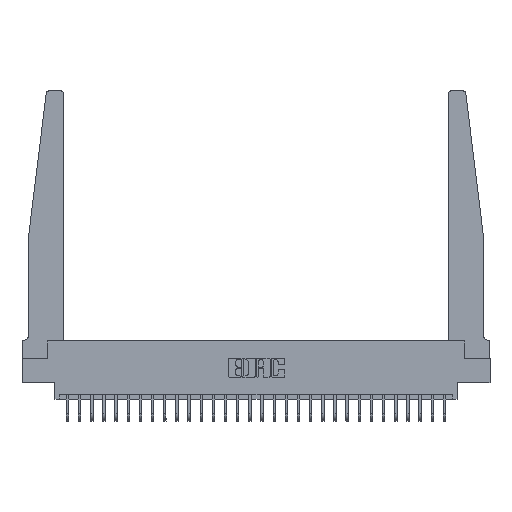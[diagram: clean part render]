
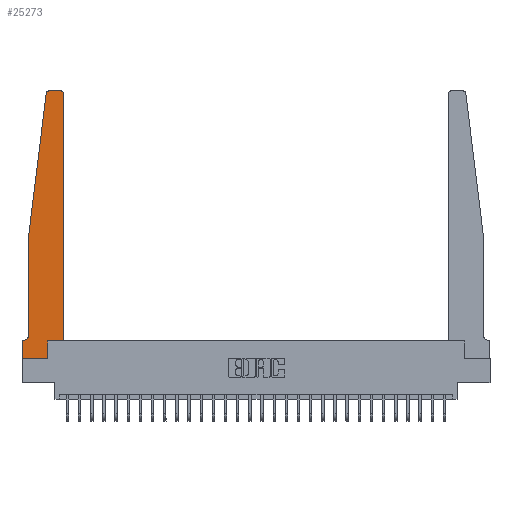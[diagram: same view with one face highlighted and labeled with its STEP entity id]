
A CAD part, top view. The second image highlights one B-rep face of the part: STEP entity #25273.
In plain terms, the highlighted planar face has unit normal (0, 0, 1).
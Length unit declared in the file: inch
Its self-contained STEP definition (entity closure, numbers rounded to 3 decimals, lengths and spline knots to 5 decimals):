
#40 = ORIENTED_EDGE ( 'NONE', *, *, #7844, .T. ) ;
#221 = VECTOR ( 'NONE', #22805, 39.37008 ) ;
#355 = EDGE_CURVE ( 'NONE', #20251, #21731, #25838, .T. ) ;
#581 = CARTESIAN_POINT ( 'NONE',  ( 0.2605, 0.18, 0.37 ) ) ;
#600 = EDGE_CURVE ( 'NONE', #10859, #20251, #25806, .T. ) ;
#1405 = VERTEX_POINT ( 'NONE', #17581 ) ;
#1529 = EDGE_CURVE ( 'NONE', #1405, #14555, #12156, .T. ) ;
#2232 = AXIS2_PLACEMENT_3D ( 'NONE', #16033, #5373, #23232 ) ;
#3076 = CARTESIAN_POINT ( 'NONE',  ( 0.24675, 2.72367, 0.37 ) ) ;
#4042 = VERTEX_POINT ( 'NONE', #8769 ) ;
#4083 = EDGE_CURVE ( 'NONE', #18692, #12985, #16721, .T. ) ;
#4384 = ORIENTED_EDGE ( 'NONE', *, *, #1529, .T. ) ;
#4479 = CARTESIAN_POINT ( 'NONE',  ( 0.425, 0.18, 0.37 ) ) ;
#4892 = CARTESIAN_POINT ( 'NONE',  ( 0.2605, 0., 0.37 ) ) ;
#5170 = DIRECTION ( 'NONE',  ( 0., -1., 0. ) ) ;
#5373 = DIRECTION ( 'NONE',  ( 0., 0., 1. ) ) ;
#6184 = ORIENTED_EDGE ( 'NONE', *, *, #24837, .T. ) ;
#6224 = DIRECTION ( 'NONE',  ( -1., 0., 0. ) ) ;
#6511 = VERTEX_POINT ( 'NONE', #16895 ) ;
#6573 = AXIS2_PLACEMENT_3D ( 'NONE', #20766, #27354, #16275 ) ;
#6804 = EDGE_CURVE ( 'NONE', #14555, #16537, #26115, .T. ) ;
#7166 = CARTESIAN_POINT ( 'NONE',  ( 0.25, 2.75, 0.37 ) ) ;
#7397 = CARTESIAN_POINT ( 'NONE',  ( 0., 0.1875, 0.37 ) ) ;
#7461 = CARTESIAN_POINT ( 'NONE',  ( 0., 0.1875, 0.37 ) ) ;
#7844 = EDGE_CURVE ( 'NONE', #16537, #6511, #19472, .T. ) ;
#8006 = VECTOR ( 'NONE', #6224, 39.37008 ) ;
#8361 = CARTESIAN_POINT ( 'NONE',  ( 0.425, 0.18, 0.37 ) ) ;
#8573 = CARTESIAN_POINT ( 'NONE',  ( 0.065, 1.25, 0.37 ) ) ;
#8655 = CARTESIAN_POINT ( 'NONE',  ( 0.425, 2.72, 0.37 ) ) ;
#8769 = CARTESIAN_POINT ( 'NONE',  ( 0.015, 0.1875, 0.37 ) ) ;
#10547 = CIRCLE ( 'NONE', #6573, 0.03 ) ;
#10859 = VERTEX_POINT ( 'NONE', #24027 ) ;
#10889 = CARTESIAN_POINT ( 'NONE',  ( 0.2605, 0.18, 0.37 ) ) ;
#10948 = CIRCLE ( 'NONE', #21295, 0.05 ) ;
#11632 = CARTESIAN_POINT ( 'NONE',  ( 0.425, 0.18, 0.37 ) ) ;
#11810 = DIRECTION ( 'NONE',  ( 1., 0., 0. ) ) ;
#12156 = LINE ( 'NONE', #7166, #221 ) ;
#12752 = VERTEX_POINT ( 'NONE', #17299 ) ;
#12789 = CARTESIAN_POINT ( 'NONE',  ( 0., 0., 0.37 ) ) ;
#12831 = CARTESIAN_POINT ( 'NONE',  ( 0.065, 1.25, 0.37 ) ) ;
#12841 = EDGE_CURVE ( 'NONE', #4042, #27306, #12900, .T. ) ;
#12900 = LINE ( 'NONE', #21653, #8006 ) ;
#12985 = VERTEX_POINT ( 'NONE', #8655 ) ;
#13246 = VECTOR ( 'NONE', #5170, 39.37008 ) ;
#13270 = VECTOR ( 'NONE', #14300, 39.37008 ) ;
#13474 = PLANE ( 'NONE',  #16370 ) ;
#13903 = ORIENTED_EDGE ( 'NONE', *, *, #600, .T. ) ;
#14239 = VECTOR ( 'NONE', #24828, 39.37008 ) ;
#14300 = DIRECTION ( 'NONE',  ( 0., 1., 0. ) ) ;
#14555 = VERTEX_POINT ( 'NONE', #26688 ) ;
#14816 = CARTESIAN_POINT ( 'NONE',  ( 0.015, 0.2375, 0.37 ) ) ;
#14996 = DIRECTION ( 'NONE',  ( 0., -1., 0. ) ) ;
#15184 = VECTOR ( 'NONE', #14996, 39.37008 ) ;
#16033 = CARTESIAN_POINT ( 'NONE',  ( 0.27653, 2.72, 0.37 ) ) ;
#16275 = DIRECTION ( 'NONE',  ( 1., 0., 0. ) ) ;
#16370 = AXIS2_PLACEMENT_3D ( 'NONE', #7397, #20832, #11810 ) ;
#16371 = ORIENTED_EDGE ( 'NONE', *, *, #28558, .T. ) ;
#16537 = VERTEX_POINT ( 'NONE', #3076 ) ;
#16721 = LINE ( 'NONE', #4479, #14239 ) ;
#16723 = EDGE_CURVE ( 'NONE', #6511, #12752, #16950, .T. ) ;
#16852 = LINE ( 'NONE', #8361, #18947 ) ;
#16895 = CARTESIAN_POINT ( 'NONE',  ( 0.065, 1.25, 0.37 ) ) ;
#16950 = LINE ( 'NONE', #12831, #15184 ) ;
#17299 = CARTESIAN_POINT ( 'NONE',  ( 0.065, 0.2375, 0.37 ) ) ;
#17499 = DIRECTION ( 'NONE',  ( 1., 0., 0. ) ) ;
#17581 = CARTESIAN_POINT ( 'NONE',  ( 0.395, 2.75, 0.37 ) ) ;
#18186 = VECTOR ( 'NONE', #19662, 39.37008 ) ;
#18450 = VECTOR ( 'NONE', #24270, 39.37008 ) ;
#18692 = VERTEX_POINT ( 'NONE', #11632 ) ;
#18947 = VECTOR ( 'NONE', #17499, 39.37008 ) ;
#19472 = LINE ( 'NONE', #8573, #18450 ) ;
#19609 = ORIENTED_EDGE ( 'NONE', *, *, #16723, .T. ) ;
#19662 = DIRECTION ( 'NONE',  ( 1., 0., 0. ) ) ;
#20251 = VERTEX_POINT ( 'NONE', #4892 ) ;
#20695 = ORIENTED_EDGE ( 'NONE', *, *, #355, .T. ) ;
#20766 = CARTESIAN_POINT ( 'NONE',  ( 0.395, 2.72, 0.37 ) ) ;
#20832 = DIRECTION ( 'NONE',  ( 0., 0., 1. ) ) ;
#21295 = AXIS2_PLACEMENT_3D ( 'NONE', #14816, #26279, #28240 ) ;
#21642 = EDGE_CURVE ( 'NONE', #12752, #4042, #10948, .T. ) ;
#21653 = CARTESIAN_POINT ( 'NONE',  ( 0.065, 0.1875, 0.37 ) ) ;
#21731 = VERTEX_POINT ( 'NONE', #10889 ) ;
#22186 = ORIENTED_EDGE ( 'NONE', *, *, #6804, .T. ) ;
#22271 = FACE_OUTER_BOUND ( 'NONE', #24308, .T. ) ;
#22805 = DIRECTION ( 'NONE',  ( -1., 0., 0. ) ) ;
#23048 = ORIENTED_EDGE ( 'NONE', *, *, #4083, .T. ) ;
#23232 = DIRECTION ( 'NONE',  ( 1., 0., 0. ) ) ;
#23773 = EDGE_CURVE ( 'NONE', #21731, #18692, #16852, .T. ) ;
#24027 = CARTESIAN_POINT ( 'NONE',  ( 0., 0., 0.37 ) ) ;
#24270 = DIRECTION ( 'NONE',  ( -0.122, -0.992, 0. ) ) ;
#24308 = EDGE_LOOP ( 'NONE', ( #4384, #22186, #40, #19609, #24866, #28657, #6184, #13903, #20695, #27128, #23048, #16371 ) ) ;
#24828 = DIRECTION ( 'NONE',  ( 0., 1., 0. ) ) ;
#24837 = EDGE_CURVE ( 'NONE', #27306, #10859, #28569, .T. ) ;
#24842 = CARTESIAN_POINT ( 'NONE',  ( 0., 0., 0.37 ) ) ;
#24866 = ORIENTED_EDGE ( 'NONE', *, *, #21642, .T. ) ;
#25273 = ADVANCED_FACE ( 'NONE', ( #22271 ), #13474, .T. ) ;
#25806 = LINE ( 'NONE', #12789, #18186 ) ;
#25838 = LINE ( 'NONE', #581, #13270 ) ;
#26115 = CIRCLE ( 'NONE', #2232, 0.03 ) ;
#26279 = DIRECTION ( 'NONE',  ( 0., 0., -1. ) ) ;
#26688 = CARTESIAN_POINT ( 'NONE',  ( 0.27653, 2.75, 0.37 ) ) ;
#27128 = ORIENTED_EDGE ( 'NONE', *, *, #23773, .T. ) ;
#27306 = VERTEX_POINT ( 'NONE', #7461 ) ;
#27354 = DIRECTION ( 'NONE',  ( 0., 0., 1. ) ) ;
#28240 = DIRECTION ( 'NONE',  ( -1., 0., 0. ) ) ;
#28558 = EDGE_CURVE ( 'NONE', #12985, #1405, #10547, .T. ) ;
#28569 = LINE ( 'NONE', #24842, #13246 ) ;
#28657 = ORIENTED_EDGE ( 'NONE', *, *, #12841, .T. ) ;
